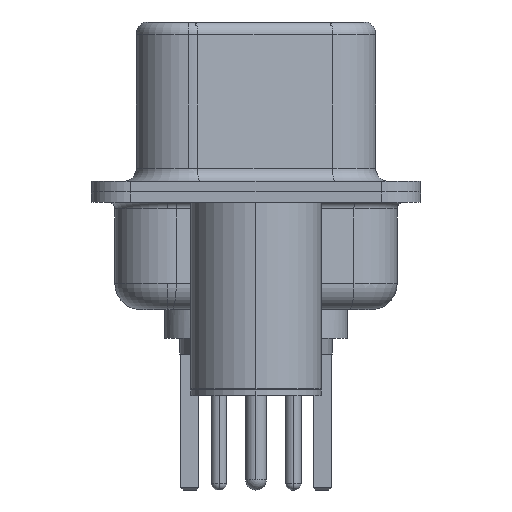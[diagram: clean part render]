
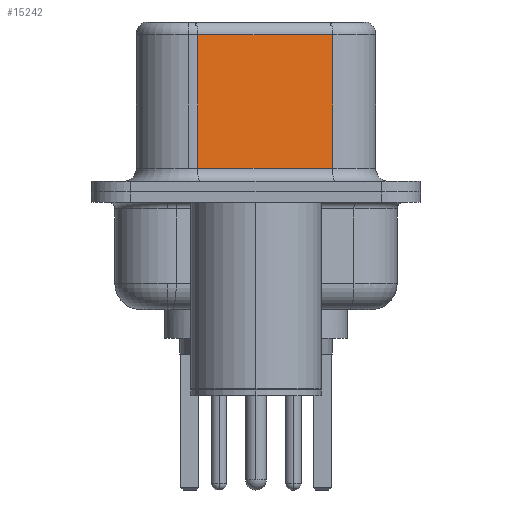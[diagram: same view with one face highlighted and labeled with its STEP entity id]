
A CAD part, left-side view. The second image highlights one B-rep face of the part: STEP entity #15242.
In plain terms, the highlighted planar face has unit normal (-0.985, -0.174, 0).
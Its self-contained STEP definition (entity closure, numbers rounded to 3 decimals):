
#560 = ORIENTED_EDGE ( 'NONE', *, *, #16423, .T. ) ;
#1822 = CARTESIAN_POINT ( 'NONE',  ( 4.58, -2.927, 6.52 ) ) ;
#2513 = LINE ( 'NONE', #4820, #13181 ) ;
#2703 = VECTOR ( 'NONE', #3787, 1000. ) ;
#3787 = DIRECTION ( 'NONE',  ( 0.174, -0.985, 0. ) ) ;
#4215 = EDGE_CURVE ( 'NONE', #23514, #24912, #4848, .T. ) ;
#4820 = CARTESIAN_POINT ( 'NONE',  ( 3.67, 2.233, 6.52 ) ) ;
#4848 = LINE ( 'NONE', #25677, #20266 ) ;
#5275 = EDGE_LOOP ( 'NONE', ( #11793, #560, #18618, #14772 ) ) ;
#5391 = FACE_OUTER_BOUND ( 'NONE', #5275, .T. ) ;
#5704 = PLANE ( 'NONE',  #9740 ) ;
#6832 = DIRECTION ( 'NONE',  ( 0., 0., -1. ) ) ;
#7681 = VERTEX_POINT ( 'NONE', #11148 ) ;
#7985 = DIRECTION ( 'NONE',  ( 0., 0., -1. ) ) ;
#9740 = AXIS2_PLACEMENT_3D ( 'NONE', #1822, #21944, #9838 ) ;
#9838 = DIRECTION ( 'NONE',  ( -0.174, 0.985, 0. ) ) ;
#9880 = LINE ( 'NONE', #17768, #2703 ) ;
#10658 = CARTESIAN_POINT ( 'NONE',  ( 4.58, -2.927, 6.02 ) ) ;
#11148 = CARTESIAN_POINT ( 'NONE',  ( 3.67, 2.233, 0.9 ) ) ;
#11793 = ORIENTED_EDGE ( 'NONE', *, *, #4215, .F. ) ;
#12679 = DIRECTION ( 'NONE',  ( -0.174, 0.985, 0. ) ) ;
#12932 = VECTOR ( 'NONE', #12679, 1000. ) ;
#13181 = VECTOR ( 'NONE', #6832, 1000. ) ;
#14772 = ORIENTED_EDGE ( 'NONE', *, *, #21745, .T. ) ;
#15242 = ADVANCED_FACE ( 'NONE', ( #5391 ), #5704, .F. ) ;
#16423 = EDGE_CURVE ( 'NONE', #23514, #22114, #18878, .T. ) ;
#16623 = CARTESIAN_POINT ( 'NONE',  ( 4.58, -2.927, 0.9 ) ) ;
#16696 = CARTESIAN_POINT ( 'NONE',  ( 3.67, 2.233, 6.02 ) ) ;
#17768 = CARTESIAN_POINT ( 'NONE',  ( 4.58, -2.927, 0.9 ) ) ;
#18279 = EDGE_CURVE ( 'NONE', #22114, #7681, #2513, .T. ) ;
#18618 = ORIENTED_EDGE ( 'NONE', *, *, #18279, .T. ) ;
#18878 = LINE ( 'NONE', #10658, #12932 ) ;
#19725 = CARTESIAN_POINT ( 'NONE',  ( 4.58, -2.927, 6.02 ) ) ;
#20266 = VECTOR ( 'NONE', #7985, 1000. ) ;
#21745 = EDGE_CURVE ( 'NONE', #7681, #24912, #9880, .T. ) ;
#21944 = DIRECTION ( 'NONE',  ( 0.985, 0.174, 0. ) ) ;
#22114 = VERTEX_POINT ( 'NONE', #16696 ) ;
#23514 = VERTEX_POINT ( 'NONE', #19725 ) ;
#24912 = VERTEX_POINT ( 'NONE', #16623 ) ;
#25677 = CARTESIAN_POINT ( 'NONE',  ( 4.58, -2.927, 6.52 ) ) ;
